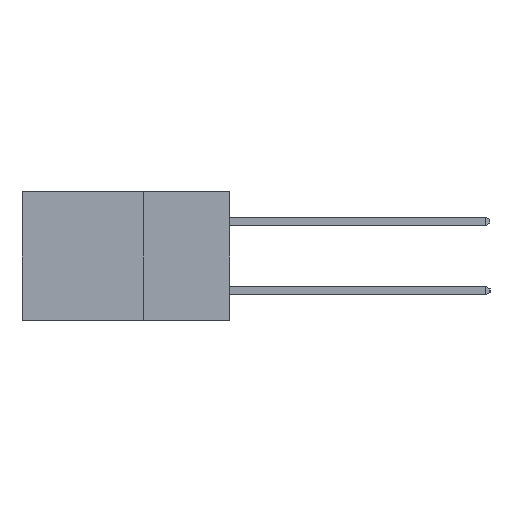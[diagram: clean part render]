
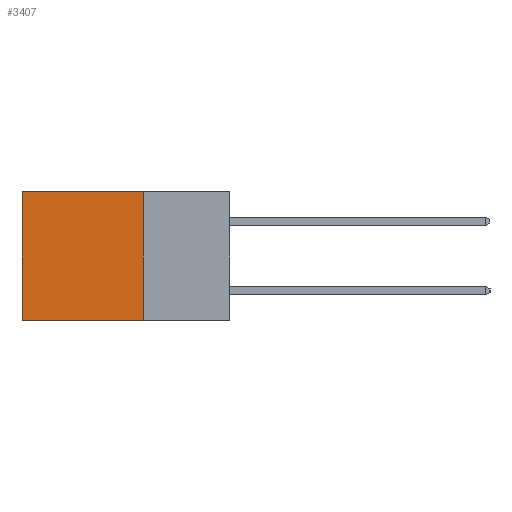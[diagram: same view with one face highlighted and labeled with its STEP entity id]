
A CAD part, left-side view. The second image highlights one B-rep face of the part: STEP entity #3407.
In plain terms, the highlighted planar face has unit normal (-1, 0, 0).
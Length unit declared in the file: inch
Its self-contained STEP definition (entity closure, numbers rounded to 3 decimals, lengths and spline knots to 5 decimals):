
#1863 = LINE ( 'NONE', #5389, #14807 ) ;
#2010 = CARTESIAN_POINT ( 'NONE',  ( 0.2615, 0.25, 0. ) ) ;
#2324 = ORIENTED_EDGE ( 'NONE', *, *, #15656, .F. ) ;
#2721 = AXIS2_PLACEMENT_3D ( 'NONE', #12410, #12239, #12184 ) ;
#3407 = ADVANCED_FACE ( 'NONE', ( #14196 ), #12513, .F. ) ;
#3512 = LINE ( 'NONE', #4014, #10033 ) ;
#3678 = LINE ( 'NONE', #8359, #4079 ) ;
#4014 = CARTESIAN_POINT ( 'NONE',  ( 0.2615, 0.25, -0.37 ) ) ;
#4079 = VECTOR ( 'NONE', #8728, 39.37008 ) ;
#4570 = VERTEX_POINT ( 'NONE', #9563 ) ;
#4606 = EDGE_CURVE ( 'NONE', #8822, #7780, #3678, .T. ) ;
#4626 = VERTEX_POINT ( 'NONE', #8107 ) ;
#5389 = CARTESIAN_POINT ( 'NONE',  ( 0.2615, 0.25, -0.37 ) ) ;
#6430 = ORIENTED_EDGE ( 'NONE', *, *, #4606, .T. ) ;
#6696 = VECTOR ( 'NONE', #16128, 39.37008 ) ;
#7496 = EDGE_CURVE ( 'NONE', #4626, #8822, #13501, .T. ) ;
#7716 = EDGE_CURVE ( 'NONE', #4570, #7780, #3512, .T. ) ;
#7780 = VERTEX_POINT ( 'NONE', #10451 ) ;
#8107 = CARTESIAN_POINT ( 'NONE',  ( 0.2615, 0.25, 0. ) ) ;
#8359 = CARTESIAN_POINT ( 'NONE',  ( 0.2615, 0.6, -0.37 ) ) ;
#8728 = DIRECTION ( 'NONE',  ( 0., 0., -1. ) ) ;
#8822 = VERTEX_POINT ( 'NONE', #10006 ) ;
#9563 = CARTESIAN_POINT ( 'NONE',  ( 0.2615, 0.25, -0.37 ) ) ;
#10006 = CARTESIAN_POINT ( 'NONE',  ( 0.2615, 0.6, 0. ) ) ;
#10033 = VECTOR ( 'NONE', #14322, 39.37008 ) ;
#10451 = CARTESIAN_POINT ( 'NONE',  ( 0.2615, 0.6, -0.37 ) ) ;
#10787 = EDGE_LOOP ( 'NONE', ( #6430, #11661, #2324, #16186 ) ) ;
#11661 = ORIENTED_EDGE ( 'NONE', *, *, #7716, .F. ) ;
#12184 = DIRECTION ( 'NONE',  ( 0., 0., -1. ) ) ;
#12239 = DIRECTION ( 'NONE',  ( 1., 0., 0. ) ) ;
#12410 = CARTESIAN_POINT ( 'NONE',  ( 0.2615, 0.25, -0.37 ) ) ;
#12513 = PLANE ( 'NONE',  #2721 ) ;
#13501 = LINE ( 'NONE', #2010, #6696 ) ;
#14196 = FACE_OUTER_BOUND ( 'NONE', #10787, .T. ) ;
#14322 = DIRECTION ( 'NONE',  ( 0., 1., 0. ) ) ;
#14807 = VECTOR ( 'NONE', #15579, 39.37008 ) ;
#15579 = DIRECTION ( 'NONE',  ( 0., 0., -1. ) ) ;
#15656 = EDGE_CURVE ( 'NONE', #4626, #4570, #1863, .T. ) ;
#16128 = DIRECTION ( 'NONE',  ( 0., 1., 0. ) ) ;
#16186 = ORIENTED_EDGE ( 'NONE', *, *, #7496, .T. ) ;
